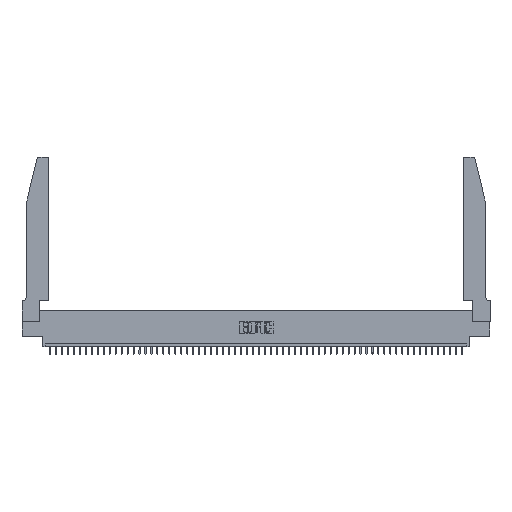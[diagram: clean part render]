
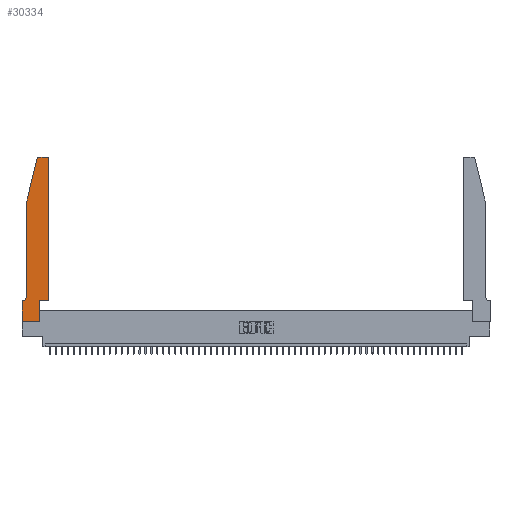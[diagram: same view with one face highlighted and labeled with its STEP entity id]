
A CAD part, top view. The second image highlights one B-rep face of the part: STEP entity #30334.
In plain terms, the highlighted planar face has unit normal (0, 0, 1).
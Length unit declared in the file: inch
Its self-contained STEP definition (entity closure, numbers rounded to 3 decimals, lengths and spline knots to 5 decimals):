
#619 = DIRECTION ( 'NONE',  ( 0., 1., 0. ) ) ;
#1036 = CARTESIAN_POINT ( 'NONE',  ( 0.4505, 2.72, 0.37 ) ) ;
#1352 = CARTESIAN_POINT ( 'NONE',  ( 0.4205, 2.72, 0.37 ) ) ;
#1696 = VECTOR ( 'NONE', #37713, 39.37008 ) ;
#1973 = DIRECTION ( 'NONE',  ( 1., 0., 0. ) ) ;
#2053 = EDGE_CURVE ( 'NONE', #29629, #44216, #20099, .T. ) ;
#2428 = CARTESIAN_POINT ( 'NONE',  ( 0.0755, 0.35, 0.37 ) ) ;
#2644 = DIRECTION ( 'NONE',  ( -0.239, -0.971, 0. ) ) ;
#2739 = CARTESIAN_POINT ( 'NONE',  ( 0.2865, 0.35, 0.37 ) ) ;
#3000 = DIRECTION ( 'NONE',  ( 0., 0., -1. ) ) ;
#3210 = CARTESIAN_POINT ( 'NONE',  ( 0., 0.35, 0.37 ) ) ;
#4529 = EDGE_CURVE ( 'NONE', #33056, #45639, #12306, .T. ) ;
#5260 = ORIENTED_EDGE ( 'NONE', *, *, #2053, .T. ) ;
#5321 = VERTEX_POINT ( 'NONE', #27090 ) ;
#8741 = VECTOR ( 'NONE', #25094, 39.37008 ) ;
#9395 = VECTOR ( 'NONE', #12023, 39.37008 ) ;
#10054 = EDGE_CURVE ( 'NONE', #31100, #34692, #11505, .T. ) ;
#10153 = LINE ( 'NONE', #18604, #51807 ) ;
#10176 = VERTEX_POINT ( 'NONE', #13652 ) ;
#10652 = DIRECTION ( 'NONE',  ( -1., 0., 0. ) ) ;
#10797 = EDGE_LOOP ( 'NONE', ( #48103, #13009, #5260, #34502, #24693, #49328, #31208, #28904, #52749, #11543, #29254, #27566 ) ) ;
#11467 = CARTESIAN_POINT ( 'NONE',  ( 0.4505, 0.35, 0.37 ) ) ;
#11505 = LINE ( 'NONE', #24317, #27376 ) ;
#11543 = ORIENTED_EDGE ( 'NONE', *, *, #31682, .T. ) ;
#12023 = DIRECTION ( 'NONE',  ( 0., -1., 0. ) ) ;
#12087 = EDGE_CURVE ( 'NONE', #52531, #29366, #31533, .T. ) ;
#12306 = CIRCLE ( 'NONE', #36615, 0.07 ) ;
#12652 = LINE ( 'NONE', #11467, #8741 ) ;
#12675 = LINE ( 'NONE', #29285, #1696 ) ;
#13009 = ORIENTED_EDGE ( 'NONE', *, *, #22135, .T. ) ;
#13619 = CARTESIAN_POINT ( 'NONE',  ( 0.25487, 2.72718, 0.37 ) ) ;
#13645 = DIRECTION ( 'NONE',  ( -1., 0., 0. ) ) ;
#13652 = CARTESIAN_POINT ( 'NONE',  ( 0., 0., 0.37 ) ) ;
#13672 = VERTEX_POINT ( 'NONE', #43543 ) ;
#13777 = CARTESIAN_POINT ( 'NONE',  ( 0.0755, 2., 0.37 ) ) ;
#14813 = VECTOR ( 'NONE', #2644, 39.37008 ) ;
#17803 = CARTESIAN_POINT ( 'NONE',  ( 0.4505, 0.35, 0.37 ) ) ;
#18357 = CARTESIAN_POINT ( 'NONE',  ( 0.284, 2.72, 0.37 ) ) ;
#18604 = CARTESIAN_POINT ( 'NONE',  ( 0., 0., 0.37 ) ) ;
#20099 = LINE ( 'NONE', #48147, #14813 ) ;
#22084 = LINE ( 'NONE', #2428, #36274 ) ;
#22135 = EDGE_CURVE ( 'NONE', #34692, #29629, #25833, .T. ) ;
#22501 = CARTESIAN_POINT ( 'NONE',  ( 0.284, 2.75, 0.37 ) ) ;
#24317 = CARTESIAN_POINT ( 'NONE',  ( 0.2605, 2.75, 0.37 ) ) ;
#24572 = AXIS2_PLACEMENT_3D ( 'NONE', #1352, #35139, #26735 ) ;
#24693 = ORIENTED_EDGE ( 'NONE', *, *, #4529, .T. ) ;
#25094 = DIRECTION ( 'NONE',  ( 1., 0., 0. ) ) ;
#25275 = EDGE_CURVE ( 'NONE', #44216, #33056, #40612, .T. ) ;
#25556 = DIRECTION ( 'NONE',  ( 0., 0., 1. ) ) ;
#25833 = CIRCLE ( 'NONE', #34521, 0.03 ) ;
#26200 = CIRCLE ( 'NONE', #24572, 0.03 ) ;
#26735 = DIRECTION ( 'NONE',  ( 1., 0., 0. ) ) ;
#27090 = CARTESIAN_POINT ( 'NONE',  ( 0., 0.35, 0.37 ) ) ;
#27248 = EDGE_CURVE ( 'NONE', #10176, #52531, #12675, .T. ) ;
#27376 = VECTOR ( 'NONE', #32467, 39.37008 ) ;
#27566 = ORIENTED_EDGE ( 'NONE', *, *, #34261, .T. ) ;
#28026 = FACE_OUTER_BOUND ( 'NONE', #10797, .T. ) ;
#28231 = VERTEX_POINT ( 'NONE', #1036 ) ;
#28377 = CARTESIAN_POINT ( 'NONE',  ( 0.0755, 2., 0.37 ) ) ;
#28478 = CARTESIAN_POINT ( 'NONE',  ( 0.0055, 0.35, 0.37 ) ) ;
#28904 = ORIENTED_EDGE ( 'NONE', *, *, #27248, .T. ) ;
#29254 = ORIENTED_EDGE ( 'NONE', *, *, #40776, .T. ) ;
#29285 = CARTESIAN_POINT ( 'NONE',  ( 0., 0., 0.37 ) ) ;
#29366 = VERTEX_POINT ( 'NONE', #2739 ) ;
#29629 = VERTEX_POINT ( 'NONE', #13619 ) ;
#30334 = ADVANCED_FACE ( 'NONE', ( #28026 ), #44618, .T. ) ;
#30867 = DIRECTION ( 'NONE',  ( 0., 0., 1. ) ) ;
#31100 = VERTEX_POINT ( 'NONE', #40389 ) ;
#31208 = ORIENTED_EDGE ( 'NONE', *, *, #39662, .T. ) ;
#31533 = LINE ( 'NONE', #35350, #41445 ) ;
#31682 = EDGE_CURVE ( 'NONE', #29366, #13672, #12652, .T. ) ;
#32467 = DIRECTION ( 'NONE',  ( -1., 0., 0. ) ) ;
#33056 = VERTEX_POINT ( 'NONE', #44364 ) ;
#34261 = EDGE_CURVE ( 'NONE', #28231, #31100, #26200, .T. ) ;
#34502 = ORIENTED_EDGE ( 'NONE', *, *, #25275, .T. ) ;
#34521 = AXIS2_PLACEMENT_3D ( 'NONE', #18357, #30867, #1973 ) ;
#34692 = VERTEX_POINT ( 'NONE', #22501 ) ;
#34729 = AXIS2_PLACEMENT_3D ( 'NONE', #3210, #25556, #42133 ) ;
#35139 = DIRECTION ( 'NONE',  ( 0., 0., 1. ) ) ;
#35350 = CARTESIAN_POINT ( 'NONE',  ( 0.2865, 0.35, 0.37 ) ) ;
#36274 = VECTOR ( 'NONE', #13645, 39.37008 ) ;
#36615 = AXIS2_PLACEMENT_3D ( 'NONE', #40048, #3000, #10652 ) ;
#37103 = VECTOR ( 'NONE', #619, 39.37008 ) ;
#37713 = DIRECTION ( 'NONE',  ( 1., 0., 0. ) ) ;
#38489 = LINE ( 'NONE', #17803, #37103 ) ;
#39662 = EDGE_CURVE ( 'NONE', #5321, #10176, #10153, .T. ) ;
#40048 = CARTESIAN_POINT ( 'NONE',  ( 0.0055, 0.42, 0.37 ) ) ;
#40389 = CARTESIAN_POINT ( 'NONE',  ( 0.4205, 2.75, 0.37 ) ) ;
#40612 = LINE ( 'NONE', #28377, #9395 ) ;
#40776 = EDGE_CURVE ( 'NONE', #13672, #28231, #38489, .T. ) ;
#41445 = VECTOR ( 'NONE', #48153, 39.37008 ) ;
#42133 = DIRECTION ( 'NONE',  ( 1., 0., 0. ) ) ;
#43500 = EDGE_CURVE ( 'NONE', #45639, #5321, #22084, .T. ) ;
#43543 = CARTESIAN_POINT ( 'NONE',  ( 0.4505, 0.35, 0.37 ) ) ;
#44216 = VERTEX_POINT ( 'NONE', #13777 ) ;
#44364 = CARTESIAN_POINT ( 'NONE',  ( 0.0755, 0.42, 0.37 ) ) ;
#44618 = PLANE ( 'NONE',  #34729 ) ;
#44781 = CARTESIAN_POINT ( 'NONE',  ( 0.2865, 0., 0.37 ) ) ;
#45639 = VERTEX_POINT ( 'NONE', #28478 ) ;
#48103 = ORIENTED_EDGE ( 'NONE', *, *, #10054, .T. ) ;
#48147 = CARTESIAN_POINT ( 'NONE',  ( 0.0755, 2., 0.37 ) ) ;
#48153 = DIRECTION ( 'NONE',  ( 0., 1., 0. ) ) ;
#49328 = ORIENTED_EDGE ( 'NONE', *, *, #43500, .T. ) ;
#51807 = VECTOR ( 'NONE', #52094, 39.37008 ) ;
#52094 = DIRECTION ( 'NONE',  ( 0., -1., 0. ) ) ;
#52531 = VERTEX_POINT ( 'NONE', #44781 ) ;
#52749 = ORIENTED_EDGE ( 'NONE', *, *, #12087, .T. ) ;
